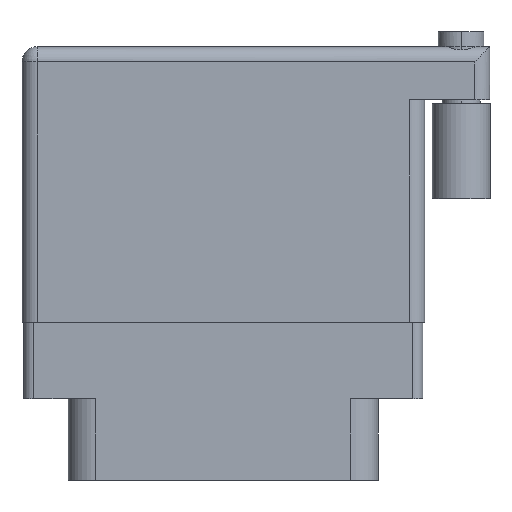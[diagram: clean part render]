
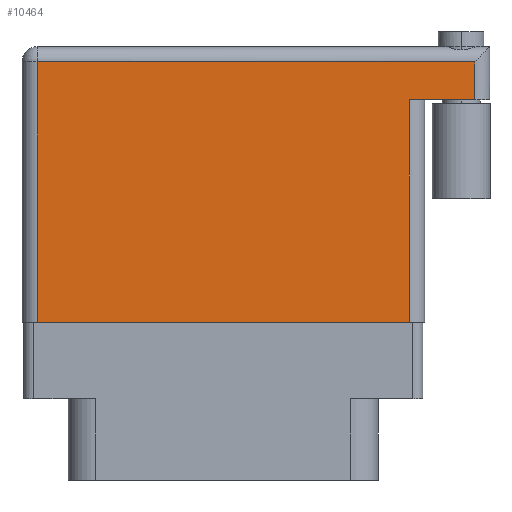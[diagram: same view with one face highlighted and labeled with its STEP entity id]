
A CAD part, front view. The second image highlights one B-rep face of the part: STEP entity #10464.
In plain terms, the highlighted face is planar.
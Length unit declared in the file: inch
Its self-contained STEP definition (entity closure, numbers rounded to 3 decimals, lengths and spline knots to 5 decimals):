
#145 = EDGE_LOOP ( 'NONE', ( #6869, #1202, #11167, #11081, #12810, #17819 ) ) ;
#273 = VERTEX_POINT ( 'NONE', #3963 ) ;
#846 = FACE_OUTER_BOUND ( 'NONE', #145, .T. ) ;
#1202 = ORIENTED_EDGE ( 'NONE', *, *, #16919, .T. ) ;
#2247 = EDGE_CURVE ( 'NONE', #2551, #14837, #15153, .T. ) ;
#2395 = EDGE_CURVE ( 'NONE', #14837, #5352, #20695, .T. ) ;
#2551 = VERTEX_POINT ( 'NONE', #18054 ) ;
#2616 = CARTESIAN_POINT ( 'NONE',  ( 0., 0.856, 0. ) ) ;
#2779 = LINE ( 'NONE', #2616, #13402 ) ;
#3813 = DIRECTION ( 'NONE',  ( 1., 0., 0. ) ) ;
#3919 = CARTESIAN_POINT ( 'NONE',  ( 1.275, 0., 0. ) ) ;
#3963 = CARTESIAN_POINT ( 'NONE',  ( 1.489, 0.856, 0. ) ) ;
#4338 = DIRECTION ( 'NONE',  ( -1., 0., 0. ) ) ;
#4928 = VERTEX_POINT ( 'NONE', #12729 ) ;
#5029 = EDGE_CURVE ( 'NONE', #273, #2551, #2779, .T. ) ;
#5352 = VERTEX_POINT ( 'NONE', #3919 ) ;
#6723 = VECTOR ( 'NONE', #19674, 39.37008 ) ;
#6869 = ORIENTED_EDGE ( 'NONE', *, *, #2395, .T. ) ;
#6891 = EDGE_CURVE ( 'NONE', #8708, #4928, #8251, .T. ) ;
#8251 = LINE ( 'NONE', #11054, #17829 ) ;
#8558 = CARTESIAN_POINT ( 'NONE',  ( 0.05, 0., 0. ) ) ;
#8708 = VERTEX_POINT ( 'NONE', #17805 ) ;
#9466 = CARTESIAN_POINT ( 'NONE',  ( 0., 0.906, 0. ) ) ;
#10124 = DIRECTION ( 'NONE',  ( 0., -1., 0. ) ) ;
#10342 = CARTESIAN_POINT ( 'NONE',  ( 0., 0., 0. ) ) ;
#10464 = ADVANCED_FACE ( 'NONE', ( #846 ), #12204, .F. ) ;
#10563 = CARTESIAN_POINT ( 'NONE',  ( 1.489, 0.906, 0. ) ) ;
#10942 = DIRECTION ( 'NONE',  ( -1., 0., 0. ) ) ;
#11054 = CARTESIAN_POINT ( 'NONE',  ( 1.539, 0.731, 0. ) ) ;
#11081 = ORIENTED_EDGE ( 'NONE', *, *, #19157, .T. ) ;
#11167 = ORIENTED_EDGE ( 'NONE', *, *, #6891, .F. ) ;
#12204 = PLANE ( 'NONE',  #15689 ) ;
#12729 = CARTESIAN_POINT ( 'NONE',  ( 1.275, 0.731, 0. ) ) ;
#12810 = ORIENTED_EDGE ( 'NONE', *, *, #5029, .T. ) ;
#13368 = CARTESIAN_POINT ( 'NONE',  ( 1.275, 0.731, 0. ) ) ;
#13402 = VECTOR ( 'NONE', #14504, 39.37008 ) ;
#14504 = DIRECTION ( 'NONE',  ( -1., 0., 0. ) ) ;
#14522 = DIRECTION ( 'NONE',  ( 0., 0., -1. ) ) ;
#14713 = LINE ( 'NONE', #10563, #6723 ) ;
#14837 = VERTEX_POINT ( 'NONE', #17107 ) ;
#15153 = LINE ( 'NONE', #8558, #18332 ) ;
#15689 = AXIS2_PLACEMENT_3D ( 'NONE', #9466, #14522, #10942 ) ;
#16438 = LINE ( 'NONE', #13368, #20383 ) ;
#16668 = DIRECTION ( 'NONE',  ( 0., 1., 0. ) ) ;
#16919 = EDGE_CURVE ( 'NONE', #5352, #4928, #16438, .T. ) ;
#17107 = CARTESIAN_POINT ( 'NONE',  ( 0.05, 0., 0. ) ) ;
#17805 = CARTESIAN_POINT ( 'NONE',  ( 1.489, 0.731, 0. ) ) ;
#17819 = ORIENTED_EDGE ( 'NONE', *, *, #2247, .T. ) ;
#17829 = VECTOR ( 'NONE', #4338, 39.37008 ) ;
#18054 = CARTESIAN_POINT ( 'NONE',  ( 0.05, 0.856, 0. ) ) ;
#18332 = VECTOR ( 'NONE', #10124, 39.37008 ) ;
#18854 = VECTOR ( 'NONE', #3813, 39.37008 ) ;
#19157 = EDGE_CURVE ( 'NONE', #8708, #273, #14713, .T. ) ;
#19674 = DIRECTION ( 'NONE',  ( 0., 1., 0. ) ) ;
#20383 = VECTOR ( 'NONE', #16668, 39.37008 ) ;
#20695 = LINE ( 'NONE', #10342, #18854 ) ;
